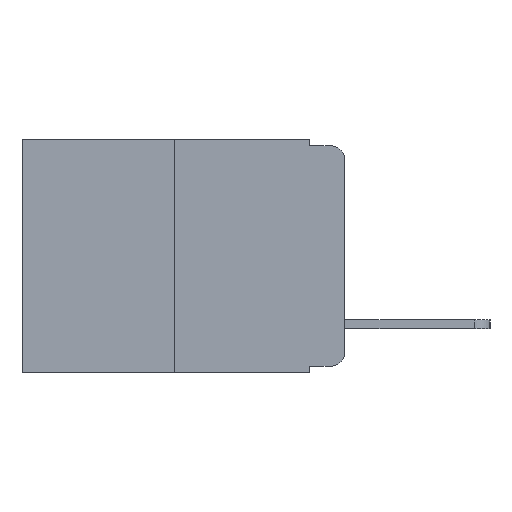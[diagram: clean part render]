
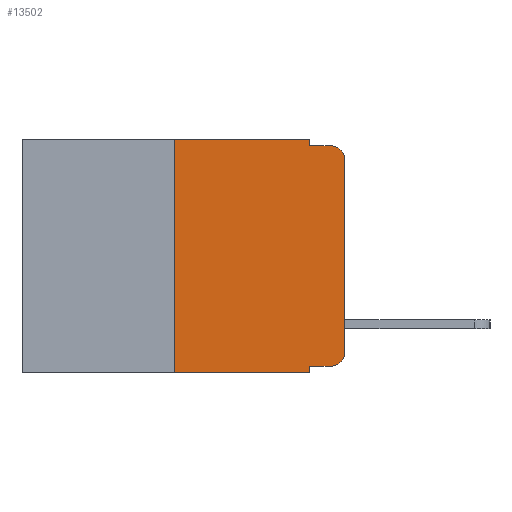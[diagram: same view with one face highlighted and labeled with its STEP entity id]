
A CAD part, left-side view. The second image highlights one B-rep face of the part: STEP entity #13502.
In plain terms, the highlighted planar face has unit normal (-1, 0, 0).
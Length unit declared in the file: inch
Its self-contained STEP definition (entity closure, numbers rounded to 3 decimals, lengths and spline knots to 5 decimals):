
#293 = DIRECTION ( 'NONE',  ( 0., -1., 0. ) ) ;
#349 = DIRECTION ( 'NONE',  ( 0., 0., -1. ) ) ;
#504 = ORIENTED_EDGE ( 'NONE', *, *, #21623, .F. ) ;
#628 = PLANE ( 'NONE',  #9504 ) ;
#2025 = ORIENTED_EDGE ( 'NONE', *, *, #8435, .F. ) ;
#2189 = VECTOR ( 'NONE', #20535, 39.37008 ) ;
#2377 = VECTOR ( 'NONE', #16226, 39.37008 ) ;
#3018 = EDGE_CURVE ( 'NONE', #19396, #5062, #22823, .T. ) ;
#3567 = CARTESIAN_POINT ( 'NONE',  ( 0., 0.473, 0. ) ) ;
#3740 = DIRECTION ( 'NONE',  ( 0., 0., -1. ) ) ;
#3794 = VERTEX_POINT ( 'NONE', #4987 ) ;
#3874 = CARTESIAN_POINT ( 'NONE',  ( 0., 0.051, -0.333 ) ) ;
#4120 = CARTESIAN_POINT ( 'NONE',  ( 0., 0.473, -0.343 ) ) ;
#4179 = EDGE_CURVE ( 'NONE', #3794, #10896, #17733, .T. ) ;
#4267 = DIRECTION ( 'NONE',  ( 0., 0., 1. ) ) ;
#4389 = EDGE_CURVE ( 'NONE', #23827, #3794, #22409, .T. ) ;
#4987 = CARTESIAN_POINT ( 'NONE',  ( 0., 0.02, -0.333 ) ) ;
#5055 = CARTESIAN_POINT ( 'NONE',  ( 0., 0., -0.313 ) ) ;
#5062 = VERTEX_POINT ( 'NONE', #18145 ) ;
#5460 = LINE ( 'NONE', #3567, #16961 ) ;
#6076 = CARTESIAN_POINT ( 'NONE',  ( 0., 0.051, 0. ) ) ;
#6217 = ORIENTED_EDGE ( 'NONE', *, *, #4389, .T. ) ;
#6282 = VECTOR ( 'NONE', #7965, 39.37008 ) ;
#6796 = ORIENTED_EDGE ( 'NONE', *, *, #10259, .T. ) ;
#6891 = LINE ( 'NONE', #4120, #6282 ) ;
#7134 = ORIENTED_EDGE ( 'NONE', *, *, #18400, .F. ) ;
#7466 = CARTESIAN_POINT ( 'NONE',  ( 0., 0.051, -0.343 ) ) ;
#7965 = DIRECTION ( 'NONE',  ( 0., -1., 0. ) ) ;
#8361 = EDGE_CURVE ( 'NONE', #17014, #19396, #17540, .T. ) ;
#8435 = EDGE_CURVE ( 'NONE', #9873, #17014, #5460, .T. ) ;
#9504 = AXIS2_PLACEMENT_3D ( 'NONE', #21735, #10369, #23608 ) ;
#9873 = VERTEX_POINT ( 'NONE', #17318 ) ;
#9924 = EDGE_CURVE ( 'NONE', #12405, #11574, #6891, .T. ) ;
#10259 = EDGE_CURVE ( 'NONE', #14694, #5062, #10724, .T. ) ;
#10369 = DIRECTION ( 'NONE',  ( 1., 0., 0. ) ) ;
#10724 = CIRCLE ( 'NONE', #17342, 0.02 ) ;
#10896 = VERTEX_POINT ( 'NONE', #5055 ) ;
#11006 = CARTESIAN_POINT ( 'NONE',  ( 0., 0.02, -0.03 ) ) ;
#11574 = VERTEX_POINT ( 'NONE', #7466 ) ;
#11718 = VECTOR ( 'NONE', #293, 39.37008 ) ;
#11972 = DIRECTION ( 'NONE',  ( -1., 0., 0. ) ) ;
#12085 = CARTESIAN_POINT ( 'NONE',  ( 0., 0.02, -0.313 ) ) ;
#12405 = VERTEX_POINT ( 'NONE', #14731 ) ;
#12972 = DIRECTION ( 'NONE',  ( 0., 0., -1. ) ) ;
#13085 = CARTESIAN_POINT ( 'NONE',  ( 0., 0.051, -0.01 ) ) ;
#13502 = ADVANCED_FACE ( 'NONE', ( #22445 ), #628, .F. ) ;
#14143 = EDGE_CURVE ( 'NONE', #10896, #14694, #22691, .T. ) ;
#14669 = AXIS2_PLACEMENT_3D ( 'NONE', #12085, #11972, #3740 ) ;
#14694 = VERTEX_POINT ( 'NONE', #19643 ) ;
#14731 = CARTESIAN_POINT ( 'NONE',  ( 0., 0.25, -0.343 ) ) ;
#14945 = DIRECTION ( 'NONE',  ( 0., -1., 0. ) ) ;
#15121 = DIRECTION ( 'NONE',  ( 0., -1., 0. ) ) ;
#15549 = CARTESIAN_POINT ( 'NONE',  ( 0., 0.051, -0.01 ) ) ;
#15785 = CARTESIAN_POINT ( 'NONE',  ( 0., 0.051, -0.333 ) ) ;
#16101 = EDGE_LOOP ( 'NONE', ( #21483, #6796, #18253, #16215, #2025, #7134, #17977, #504, #6217, #16524 ) ) ;
#16215 = ORIENTED_EDGE ( 'NONE', *, *, #8361, .F. ) ;
#16226 = DIRECTION ( 'NONE',  ( 0., 0., 1. ) ) ;
#16524 = ORIENTED_EDGE ( 'NONE', *, *, #4179, .T. ) ;
#16670 = VECTOR ( 'NONE', #349, 39.37008 ) ;
#16961 = VECTOR ( 'NONE', #15121, 39.37008 ) ;
#17014 = VERTEX_POINT ( 'NONE', #17421 ) ;
#17318 = CARTESIAN_POINT ( 'NONE',  ( 0., 0.25, 0. ) ) ;
#17342 = AXIS2_PLACEMENT_3D ( 'NONE', #11006, #24224, #12972 ) ;
#17421 = CARTESIAN_POINT ( 'NONE',  ( 0., 0.051, 0. ) ) ;
#17540 = LINE ( 'NONE', #20456, #2189 ) ;
#17705 = CARTESIAN_POINT ( 'NONE',  ( 0., 0.25, 0. ) ) ;
#17733 = CIRCLE ( 'NONE', #14669, 0.02 ) ;
#17850 = VECTOR ( 'NONE', #14945, 39.37008 ) ;
#17972 = VECTOR ( 'NONE', #4267, 39.37008 ) ;
#17977 = ORIENTED_EDGE ( 'NONE', *, *, #9924, .T. ) ;
#18145 = CARTESIAN_POINT ( 'NONE',  ( 0., 0.02, -0.01 ) ) ;
#18253 = ORIENTED_EDGE ( 'NONE', *, *, #3018, .F. ) ;
#18400 = EDGE_CURVE ( 'NONE', #12405, #9873, #23523, .T. ) ;
#19396 = VERTEX_POINT ( 'NONE', #13085 ) ;
#19643 = CARTESIAN_POINT ( 'NONE',  ( 0., 0., -0.03 ) ) ;
#19896 = CARTESIAN_POINT ( 'NONE',  ( 0., 0., 0. ) ) ;
#20456 = CARTESIAN_POINT ( 'NONE',  ( 0., 0.051, 0. ) ) ;
#20535 = DIRECTION ( 'NONE',  ( 0., 0., -1. ) ) ;
#21483 = ORIENTED_EDGE ( 'NONE', *, *, #14143, .T. ) ;
#21623 = EDGE_CURVE ( 'NONE', #23827, #11574, #21645, .T. ) ;
#21645 = LINE ( 'NONE', #6076, #16670 ) ;
#21735 = CARTESIAN_POINT ( 'NONE',  ( 0., 0.473, 0. ) ) ;
#22409 = LINE ( 'NONE', #3874, #11718 ) ;
#22445 = FACE_OUTER_BOUND ( 'NONE', #16101, .T. ) ;
#22691 = LINE ( 'NONE', #19896, #2377 ) ;
#22823 = LINE ( 'NONE', #15549, #17850 ) ;
#23523 = LINE ( 'NONE', #17705, #17972 ) ;
#23608 = DIRECTION ( 'NONE',  ( 0., 0., -1. ) ) ;
#23827 = VERTEX_POINT ( 'NONE', #15785 ) ;
#24224 = DIRECTION ( 'NONE',  ( -1., 0., 0. ) ) ;
